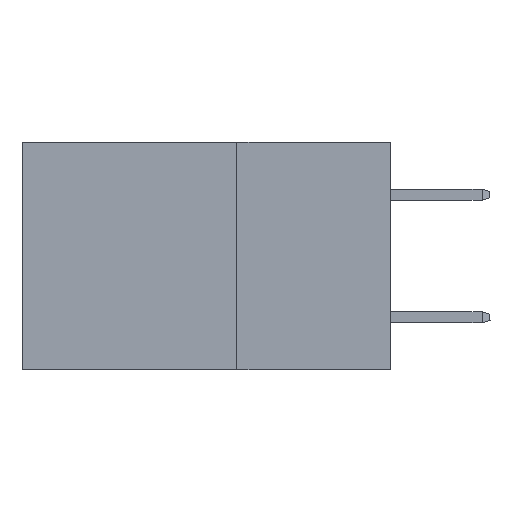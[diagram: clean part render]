
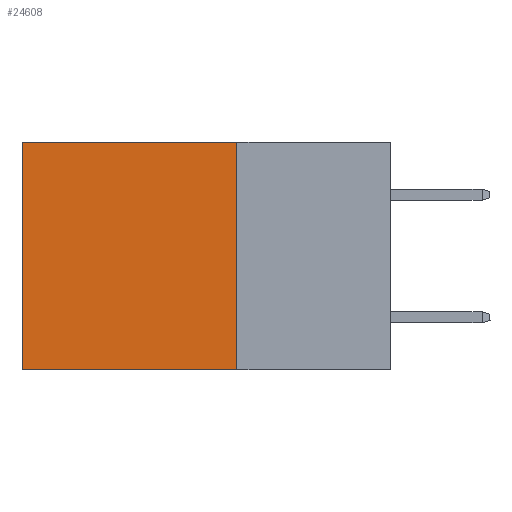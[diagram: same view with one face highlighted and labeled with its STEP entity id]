
A CAD part, left-side view. The second image highlights one B-rep face of the part: STEP entity #24608.
In plain terms, the highlighted planar face has unit normal (-1, 0, 0).
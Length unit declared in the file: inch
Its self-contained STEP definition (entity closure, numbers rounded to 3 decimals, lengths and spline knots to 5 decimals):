
#157 = VERTEX_POINT ( 'NONE', #23235 ) ;
#183 = ORIENTED_EDGE ( 'NONE', *, *, #32453, .T. ) ;
#1004 = CARTESIAN_POINT ( 'NONE',  ( 0.2875, 0.25, 0. ) ) ;
#1978 = VECTOR ( 'NONE', #24637, 39.37008 ) ;
#2175 = EDGE_CURVE ( 'NONE', #24956, #157, #24071, .T. ) ;
#3218 = AXIS2_PLACEMENT_3D ( 'NONE', #1004, #21426, #14037 ) ;
#3699 = ORIENTED_EDGE ( 'NONE', *, *, #18122, .F. ) ;
#4873 = CARTESIAN_POINT ( 'NONE',  ( 0.2875, 0.6, 0. ) ) ;
#5749 = CARTESIAN_POINT ( 'NONE',  ( 0.2875, 0.6, 0. ) ) ;
#6243 = PLANE ( 'NONE',  #3218 ) ;
#9246 = CARTESIAN_POINT ( 'NONE',  ( 0.2875, 0.25, 0. ) ) ;
#10065 = CARTESIAN_POINT ( 'NONE',  ( 0.2875, 0.25, -0.37 ) ) ;
#10182 = LINE ( 'NONE', #14817, #16221 ) ;
#12540 = VERTEX_POINT ( 'NONE', #4873 ) ;
#14037 = DIRECTION ( 'NONE',  ( 0., 0., -1. ) ) ;
#14817 = CARTESIAN_POINT ( 'NONE',  ( 0.2875, 0.25, 0. ) ) ;
#15768 = LINE ( 'NONE', #19336, #1978 ) ;
#16221 = VECTOR ( 'NONE', #20506, 39.37008 ) ;
#17164 = VECTOR ( 'NONE', #25424, 39.37008 ) ;
#17492 = CARTESIAN_POINT ( 'NONE',  ( 0.2875, 0.25, -0.37 ) ) ;
#18122 = EDGE_CURVE ( 'NONE', #20604, #24956, #15768, .T. ) ;
#18459 = DIRECTION ( 'NONE',  ( 0., 0., -1. ) ) ;
#19204 = EDGE_CURVE ( 'NONE', #12540, #157, #24236, .T. ) ;
#19336 = CARTESIAN_POINT ( 'NONE',  ( 0.2875, 0.25, 0. ) ) ;
#19525 = ORIENTED_EDGE ( 'NONE', *, *, #2175, .F. ) ;
#19984 = ORIENTED_EDGE ( 'NONE', *, *, #19204, .T. ) ;
#20506 = DIRECTION ( 'NONE',  ( 0., 1., 0. ) ) ;
#20604 = VERTEX_POINT ( 'NONE', #9246 ) ;
#21426 = DIRECTION ( 'NONE',  ( 1., 0., 0. ) ) ;
#21516 = FACE_OUTER_BOUND ( 'NONE', #27697, .T. ) ;
#23235 = CARTESIAN_POINT ( 'NONE',  ( 0.2875, 0.6, -0.37 ) ) ;
#24071 = LINE ( 'NONE', #17492, #17164 ) ;
#24236 = LINE ( 'NONE', #5749, #29992 ) ;
#24608 = ADVANCED_FACE ( 'NONE', ( #21516 ), #6243, .F. ) ;
#24637 = DIRECTION ( 'NONE',  ( 0., 0., -1. ) ) ;
#24956 = VERTEX_POINT ( 'NONE', #10065 ) ;
#25424 = DIRECTION ( 'NONE',  ( 0., 1., 0. ) ) ;
#27697 = EDGE_LOOP ( 'NONE', ( #19984, #19525, #3699, #183 ) ) ;
#29992 = VECTOR ( 'NONE', #18459, 39.37008 ) ;
#32453 = EDGE_CURVE ( 'NONE', #20604, #12540, #10182, .T. ) ;
